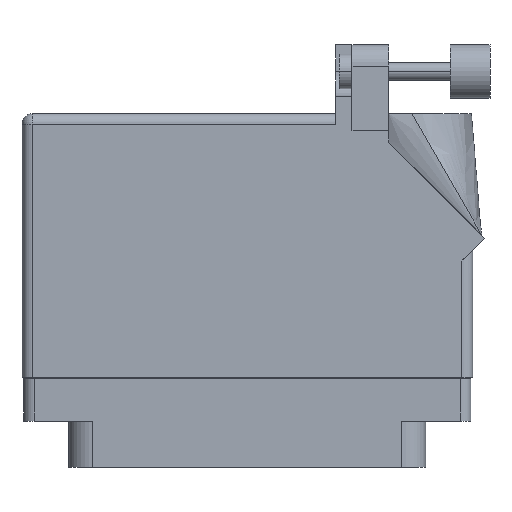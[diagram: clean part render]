
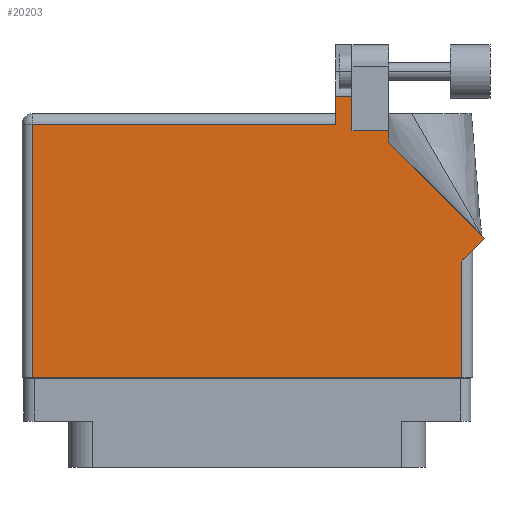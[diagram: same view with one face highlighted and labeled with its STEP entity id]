
A CAD part, front view. The second image highlights one B-rep face of the part: STEP entity #20203.
In plain terms, the highlighted face is planar.
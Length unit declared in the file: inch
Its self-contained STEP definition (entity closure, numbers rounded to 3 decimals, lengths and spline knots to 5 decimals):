
#175 = PLANE ( 'NONE',  #22666 ) ;
#690 = EDGE_CURVE ( 'NONE', #12945, #10442, #28585, .T. ) ;
#877 = ORIENTED_EDGE ( 'NONE', *, *, #34008, .T. ) ;
#932 = CARTESIAN_POINT ( 'NONE',  ( 0.82, 1.26442, 0.455 ) ) ;
#987 = ORIENTED_EDGE ( 'NONE', *, *, #4914, .T. ) ;
#1184 = EDGE_CURVE ( 'NONE', #9233, #38335, #31452, .T. ) ;
#3350 = CARTESIAN_POINT ( 'NONE',  ( 0.513, 1.43, 0.455 ) ) ;
#3487 = VECTOR ( 'NONE', #38791, 39.37008 ) ;
#3692 = VECTOR ( 'NONE', #17079, 39.37008 ) ;
#4190 = CARTESIAN_POINT ( 'NONE',  ( 0.513, 1.368, 0.455 ) ) ;
#4317 = FACE_OUTER_BOUND ( 'NONE', #4448, .T. ) ;
#4448 = EDGE_LOOP ( 'NONE', ( #10741, #11327, #18816, #35124, #877, #987, #21226, #17731, #37725, #14031, #15910 ) ) ;
#4914 = EDGE_CURVE ( 'NONE', #17007, #47682, #9238, .T. ) ;
#5504 = VERTEX_POINT ( 'NONE', #25725 ) ;
#6342 = VECTOR ( 'NONE', #34803, 39.37008 ) ;
#7818 = LINE ( 'NONE', #22693, #44318 ) ;
#9056 = VECTOR ( 'NONE', #28527, 39.37008 ) ;
#9225 = VERTEX_POINT ( 'NONE', #4190 ) ;
#9233 = VERTEX_POINT ( 'NONE', #23175 ) ;
#9238 = LINE ( 'NONE', #24102, #33759 ) ;
#10442 = VERTEX_POINT ( 'NONE', #16971 ) ;
#10741 = ORIENTED_EDGE ( 'NONE', *, *, #16779, .T. ) ;
#11327 = ORIENTED_EDGE ( 'NONE', *, *, #690, .T. ) ;
#12476 = CARTESIAN_POINT ( 'NONE',  ( 1.306, 0.637, 0.455 ) ) ;
#12945 = VERTEX_POINT ( 'NONE', #31566 ) ;
#13789 = EDGE_CURVE ( 'NONE', #30915, #35936, #27564, .T. ) ;
#13839 = CARTESIAN_POINT ( 'NONE',  ( -1.244, -0.1, 0.455 ) ) ;
#14031 = ORIENTED_EDGE ( 'NONE', *, *, #36559, .T. ) ;
#15072 = VERTEX_POINT ( 'NONE', #31703 ) ;
#15855 = DIRECTION ( 'NONE',  ( 0., 1., 0. ) ) ;
#15910 = ORIENTED_EDGE ( 'NONE', *, *, #1184, .T. ) ;
#16187 = LINE ( 'NONE', #24621, #42202 ) ;
#16779 = EDGE_CURVE ( 'NONE', #38335, #12945, #7818, .T. ) ;
#16971 = CARTESIAN_POINT ( 'NONE',  ( 0.513, 1.5315, 0.455 ) ) ;
#17007 = VERTEX_POINT ( 'NONE', #13839 ) ;
#17029 = LINE ( 'NONE', #45774, #30646 ) ;
#17079 = DIRECTION ( 'NONE',  ( 0., 1., 0. ) ) ;
#17731 = ORIENTED_EDGE ( 'NONE', *, *, #13789, .T. ) ;
#18209 = CARTESIAN_POINT ( 'NONE',  ( 1.244, -0.1, 0.455 ) ) ;
#18816 = ORIENTED_EDGE ( 'NONE', *, *, #38590, .T. ) ;
#19184 = DIRECTION ( 'NONE',  ( 0., 0., -1. ) ) ;
#20203 = ADVANCED_FACE ( 'NONE', ( #4317 ), #175, .F. ) ;
#20347 = DIRECTION ( 'NONE',  ( 0., -1., 0. ) ) ;
#21226 = ORIENTED_EDGE ( 'NONE', *, *, #28878, .T. ) ;
#22666 = AXIS2_PLACEMENT_3D ( 'NONE', #37451, #19184, #34028 ) ;
#22693 = CARTESIAN_POINT ( 'NONE',  ( 0.607, 1.33, 0.455 ) ) ;
#23175 = CARTESIAN_POINT ( 'NONE',  ( 0.82, 1.33, 0.455 ) ) ;
#23592 = LINE ( 'NONE', #932, #6342 ) ;
#23750 = LINE ( 'NONE', #27160, #46737 ) ;
#24102 = CARTESIAN_POINT ( 'NONE',  ( -1.306, -0.1, 0.455 ) ) ;
#24621 = CARTESIAN_POINT ( 'NONE',  ( 1.37671, 0.70771, 0.455 ) ) ;
#25080 = LINE ( 'NONE', #43865, #3692 ) ;
#25725 = CARTESIAN_POINT ( 'NONE',  ( -1.244, 1.368, 0.455 ) ) ;
#26771 = VECTOR ( 'NONE', #32332, 39.37008 ) ;
#27117 = DIRECTION ( 'NONE',  ( -0.707, 0.707, 0. ) ) ;
#27160 = CARTESIAN_POINT ( 'NONE',  ( -1.244, -0.1, 0.455 ) ) ;
#27564 = LINE ( 'NONE', #12476, #3487 ) ;
#28527 = DIRECTION ( 'NONE',  ( -1., 0., 0. ) ) ;
#28585 = LINE ( 'NONE', #35430, #47182 ) ;
#28878 = EDGE_CURVE ( 'NONE', #47682, #30915, #25080, .T. ) ;
#30646 = VECTOR ( 'NONE', #35518, 39.37008 ) ;
#30915 = VERTEX_POINT ( 'NONE', #46936 ) ;
#31452 = LINE ( 'NONE', #39033, #9056 ) ;
#31566 = CARTESIAN_POINT ( 'NONE',  ( 0.607, 1.5315, 0.455 ) ) ;
#31703 = CARTESIAN_POINT ( 'NONE',  ( 0.82, 1.26442, 0.455 ) ) ;
#32332 = DIRECTION ( 'NONE',  ( 0., -1., 0. ) ) ;
#32940 = CARTESIAN_POINT ( 'NONE',  ( 1.37671, 0.70771, 0.455 ) ) ;
#33759 = VECTOR ( 'NONE', #39456, 39.37008 ) ;
#34008 = EDGE_CURVE ( 'NONE', #5504, #17007, #23750, .T. ) ;
#34028 = DIRECTION ( 'NONE',  ( -1., 0., 0. ) ) ;
#34305 = CARTESIAN_POINT ( 'NONE',  ( 0.607, 1.33, 0.455 ) ) ;
#34803 = DIRECTION ( 'NONE',  ( 0., 1., 0. ) ) ;
#35124 = ORIENTED_EDGE ( 'NONE', *, *, #38350, .T. ) ;
#35430 = CARTESIAN_POINT ( 'NONE',  ( 0.93777, 1.5315, 0.455 ) ) ;
#35518 = DIRECTION ( 'NONE',  ( -1., 0., 0. ) ) ;
#35936 = VERTEX_POINT ( 'NONE', #32940 ) ;
#36559 = EDGE_CURVE ( 'NONE', #15072, #9233, #23592, .T. ) ;
#37451 = CARTESIAN_POINT ( 'NONE',  ( -1.306, 1.43, 0.455 ) ) ;
#37725 = ORIENTED_EDGE ( 'NONE', *, *, #39273, .T. ) ;
#38335 = VERTEX_POINT ( 'NONE', #34305 ) ;
#38350 = EDGE_CURVE ( 'NONE', #9225, #5504, #17029, .T. ) ;
#38590 = EDGE_CURVE ( 'NONE', #10442, #9225, #43576, .T. ) ;
#38791 = DIRECTION ( 'NONE',  ( 0.707, 0.707, 0. ) ) ;
#39033 = CARTESIAN_POINT ( 'NONE',  ( 0.82, 1.33, 0.455 ) ) ;
#39273 = EDGE_CURVE ( 'NONE', #35936, #15072, #16187, .T. ) ;
#39456 = DIRECTION ( 'NONE',  ( 1., 0., 0. ) ) ;
#42202 = VECTOR ( 'NONE', #27117, 39.37008 ) ;
#43489 = DIRECTION ( 'NONE',  ( -1., 0., 0. ) ) ;
#43576 = LINE ( 'NONE', #3350, #26771 ) ;
#43865 = CARTESIAN_POINT ( 'NONE',  ( 1.244, 0.637, 0.455 ) ) ;
#44318 = VECTOR ( 'NONE', #15855, 39.37008 ) ;
#45774 = CARTESIAN_POINT ( 'NONE',  ( -1.306, 1.368, 0.455 ) ) ;
#46737 = VECTOR ( 'NONE', #20347, 39.37008 ) ;
#46936 = CARTESIAN_POINT ( 'NONE',  ( 1.244, 0.575, 0.455 ) ) ;
#47182 = VECTOR ( 'NONE', #43489, 39.37008 ) ;
#47682 = VERTEX_POINT ( 'NONE', #18209 ) ;
